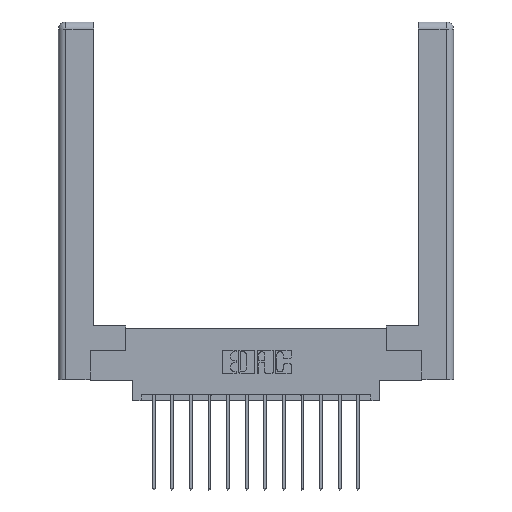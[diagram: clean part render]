
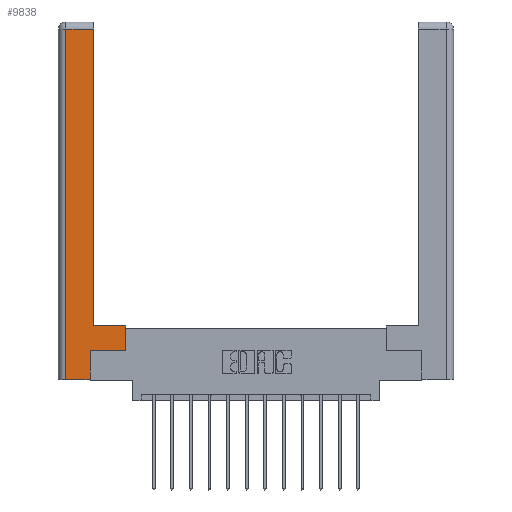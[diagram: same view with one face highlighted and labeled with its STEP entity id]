
A CAD part, top view. The second image highlights one B-rep face of the part: STEP entity #9838.
In plain terms, the highlighted planar face has unit normal (0, 0, 1).
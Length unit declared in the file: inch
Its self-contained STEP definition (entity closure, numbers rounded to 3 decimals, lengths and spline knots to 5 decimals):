
#700 = PLANE ( 'NONE',  #12321 ) ;
#847 = LINE ( 'NONE', #2498, #3020 ) ;
#1182 = CARTESIAN_POINT ( 'NONE',  ( 0.295, 0.45, 0. ) ) ;
#1334 = ORIENTED_EDGE ( 'NONE', *, *, #10288, .T. ) ;
#1571 = LINE ( 'NONE', #6741, #7374 ) ;
#1597 = VERTEX_POINT ( 'NONE', #8046 ) ;
#1840 = VECTOR ( 'NONE', #11543, 39.37008 ) ;
#2019 = FACE_OUTER_BOUND ( 'NONE', #5200, .T. ) ;
#2127 = VERTEX_POINT ( 'NONE', #15080 ) ;
#2432 = DIRECTION ( 'NONE',  ( 1., 0., 0. ) ) ;
#2498 = CARTESIAN_POINT ( 'NONE',  ( 0.265, 0., 0. ) ) ;
#2503 = ORIENTED_EDGE ( 'NONE', *, *, #6426, .T. ) ;
#2574 = DIRECTION ( 'NONE',  ( 1., 0., 0. ) ) ;
#2908 = CARTESIAN_POINT ( 'NONE',  ( 0.0615, 2.94, 0. ) ) ;
#3020 = VECTOR ( 'NONE', #2432, 39.37008 ) ;
#3131 = EDGE_CURVE ( 'NONE', #1597, #14213, #14208, .T. ) ;
#3272 = DIRECTION ( 'NONE',  ( 0., 1., 0. ) ) ;
#3794 = CARTESIAN_POINT ( 'NONE',  ( 0.565, 0.45, 0. ) ) ;
#4502 = CARTESIAN_POINT ( 'NONE',  ( 0.295, 3., 0. ) ) ;
#5200 = EDGE_LOOP ( 'NONE', ( #10167, #9611, #9341, #1334, #12556, #15938, #6051, #2503 ) ) ;
#5266 = CARTESIAN_POINT ( 'NONE',  ( 0.265, 0.245, 0. ) ) ;
#6051 = ORIENTED_EDGE ( 'NONE', *, *, #8886, .T. ) ;
#6426 = EDGE_CURVE ( 'NONE', #12831, #11142, #1571, .T. ) ;
#6741 = CARTESIAN_POINT ( 'NONE',  ( 0.295, 0.45, 0. ) ) ;
#6829 = CARTESIAN_POINT ( 'NONE',  ( 0., 0., 0. ) ) ;
#7054 = EDGE_CURVE ( 'NONE', #12848, #14267, #15069, .T. ) ;
#7090 = LINE ( 'NONE', #11855, #14251 ) ;
#7374 = VECTOR ( 'NONE', #12360, 39.37008 ) ;
#7545 = CARTESIAN_POINT ( 'NONE',  ( 0.265, 0., 0. ) ) ;
#7576 = EDGE_CURVE ( 'NONE', #11142, #1597, #10794, .T. ) ;
#7745 = DIRECTION ( 'NONE',  ( 0., 1., 0. ) ) ;
#8046 = CARTESIAN_POINT ( 'NONE',  ( 0.295, 2.94, 0. ) ) ;
#8085 = CARTESIAN_POINT ( 'NONE',  ( 0.265, 0.245, 0. ) ) ;
#8125 = CARTESIAN_POINT ( 'NONE',  ( 0.565, 0.245, 0. ) ) ;
#8128 = DIRECTION ( 'NONE',  ( 0., 1., 0. ) ) ;
#8292 = LINE ( 'NONE', #8783, #8473 ) ;
#8473 = VECTOR ( 'NONE', #2574, 39.37008 ) ;
#8783 = CARTESIAN_POINT ( 'NONE',  ( 0.565, 0.245, 0. ) ) ;
#8886 = EDGE_CURVE ( 'NONE', #9825, #12831, #7090, .T. ) ;
#9249 = DIRECTION ( 'NONE',  ( 0., 0., -1. ) ) ;
#9341 = ORIENTED_EDGE ( 'NONE', *, *, #12758, .T. ) ;
#9611 = ORIENTED_EDGE ( 'NONE', *, *, #3131, .T. ) ;
#9659 = EDGE_CURVE ( 'NONE', #14267, #9825, #8292, .T. ) ;
#9825 = VERTEX_POINT ( 'NONE', #8125 ) ;
#9838 = ADVANCED_FACE ( 'NONE', ( #2019 ), #700, .F. ) ;
#10167 = ORIENTED_EDGE ( 'NONE', *, *, #7576, .T. ) ;
#10288 = EDGE_CURVE ( 'NONE', #2127, #12848, #847, .T. ) ;
#10641 = DIRECTION ( 'NONE',  ( -1., 0., 0. ) ) ;
#10794 = LINE ( 'NONE', #4502, #12912 ) ;
#11142 = VERTEX_POINT ( 'NONE', #1182 ) ;
#11357 = VECTOR ( 'NONE', #15094, 39.37008 ) ;
#11543 = DIRECTION ( 'NONE',  ( -1., 0., 0. ) ) ;
#11746 = LINE ( 'NONE', #14922, #11357 ) ;
#11855 = CARTESIAN_POINT ( 'NONE',  ( 0.565, 0.45, 0. ) ) ;
#11857 = CARTESIAN_POINT ( 'NONE',  ( 0.0615, 2.94, 0. ) ) ;
#12321 = AXIS2_PLACEMENT_3D ( 'NONE', #6829, #9249, #10641 ) ;
#12360 = DIRECTION ( 'NONE',  ( -1., 0., 0. ) ) ;
#12556 = ORIENTED_EDGE ( 'NONE', *, *, #7054, .T. ) ;
#12758 = EDGE_CURVE ( 'NONE', #14213, #2127, #11746, .T. ) ;
#12831 = VERTEX_POINT ( 'NONE', #3794 ) ;
#12848 = VERTEX_POINT ( 'NONE', #7545 ) ;
#12912 = VECTOR ( 'NONE', #3272, 39.37008 ) ;
#13111 = VECTOR ( 'NONE', #7745, 39.37008 ) ;
#14208 = LINE ( 'NONE', #2908, #1840 ) ;
#14213 = VERTEX_POINT ( 'NONE', #11857 ) ;
#14251 = VECTOR ( 'NONE', #8128, 39.37008 ) ;
#14267 = VERTEX_POINT ( 'NONE', #8085 ) ;
#14922 = CARTESIAN_POINT ( 'NONE',  ( 0.0615, 0., 0. ) ) ;
#15069 = LINE ( 'NONE', #5266, #13111 ) ;
#15080 = CARTESIAN_POINT ( 'NONE',  ( 0.0615, 0., 0. ) ) ;
#15094 = DIRECTION ( 'NONE',  ( 0., -1., 0. ) ) ;
#15938 = ORIENTED_EDGE ( 'NONE', *, *, #9659, .T. ) ;
